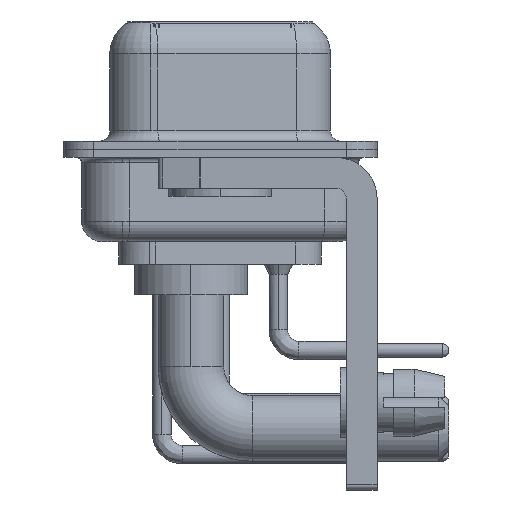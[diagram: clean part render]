
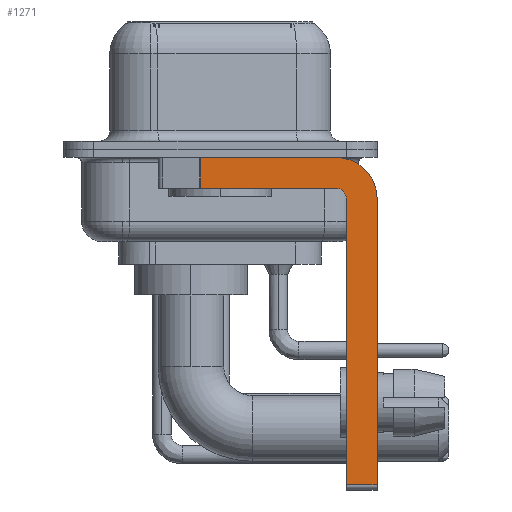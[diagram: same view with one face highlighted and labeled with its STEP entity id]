
A CAD part, left-side view. The second image highlights one B-rep face of the part: STEP entity #1271.
In plain terms, the highlighted planar face has unit normal (-1, 0, 0).
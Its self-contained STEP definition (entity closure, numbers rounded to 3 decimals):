
#229 = ORIENTED_EDGE ( 'NONE', *, *, #22137, .F. ) ;
#517 = DIRECTION ( 'NONE',  ( 0., 0., 1. ) ) ;
#1271 = ADVANCED_FACE ( 'NONE', ( #22588 ), #27415, .F. ) ;
#1882 = ORIENTED_EDGE ( 'NONE', *, *, #24168, .T. ) ;
#2416 = EDGE_CURVE ( 'NONE', #10307, #3281, #25507, .T. ) ;
#2463 = DIRECTION ( 'NONE',  ( 0., 0., -1. ) ) ;
#2919 = ORIENTED_EDGE ( 'NONE', *, *, #3153, .F. ) ;
#3153 = EDGE_CURVE ( 'NONE', #4360, #13230, #18464, .T. ) ;
#3281 = VERTEX_POINT ( 'NONE', #10403 ) ;
#3462 = ORIENTED_EDGE ( 'NONE', *, *, #10106, .F. ) ;
#3526 = DIRECTION ( 'NONE',  ( -1., 0., 0. ) ) ;
#4246 = DIRECTION ( 'NONE',  ( 0., 0., -1. ) ) ;
#4360 = VERTEX_POINT ( 'NONE', #17540 ) ;
#5350 = DIRECTION ( 'NONE',  ( 0., -1., 0. ) ) ;
#5502 = VECTOR ( 'NONE', #13557, 1000. ) ;
#6138 = AXIS2_PLACEMENT_3D ( 'NONE', #22110, #17615, #10553 ) ;
#6994 = EDGE_LOOP ( 'NONE', ( #8027, #1882, #2919, #229, #3462, #15904, #24967, #16377 ) ) ;
#7611 = CARTESIAN_POINT ( 'NONE',  ( -2.9, 3., -0.4 ) ) ;
#8027 = ORIENTED_EDGE ( 'NONE', *, *, #10384, .F. ) ;
#9107 = CARTESIAN_POINT ( 'NONE',  ( -2.9, -6.15, -16.35 ) ) ;
#10106 = EDGE_CURVE ( 'NONE', #26981, #18680, #11628, .T. ) ;
#10307 = VERTEX_POINT ( 'NONE', #22043 ) ;
#10359 = EDGE_CURVE ( 'NONE', #30653, #10307, #19841, .T. ) ;
#10384 = EDGE_CURVE ( 'NONE', #18487, #30653, #17218, .T. ) ;
#10403 = CARTESIAN_POINT ( 'NONE',  ( -2.9, -7.65, -16.35 ) ) ;
#10553 = DIRECTION ( 'NONE',  ( 0., 0., -1. ) ) ;
#11628 = LINE ( 'NONE', #25754, #5502 ) ;
#13230 = VERTEX_POINT ( 'NONE', #29028 ) ;
#13351 = DIRECTION ( 'NONE',  ( 0., 1., 0. ) ) ;
#13557 = DIRECTION ( 'NONE',  ( 0., 0., 1. ) ) ;
#15904 = ORIENTED_EDGE ( 'NONE', *, *, #20538, .T. ) ;
#16348 = CARTESIAN_POINT ( 'NONE',  ( -2.9, -7.65, -2.4 ) ) ;
#16377 = ORIENTED_EDGE ( 'NONE', *, *, #10359, .F. ) ;
#16552 = LINE ( 'NONE', #26031, #20680 ) ;
#16585 = VECTOR ( 'NONE', #13351, 1000. ) ;
#16738 = CARTESIAN_POINT ( 'NONE',  ( -2.9, -5.65, -2.4 ) ) ;
#17218 = LINE ( 'NONE', #7611, #27044 ) ;
#17540 = CARTESIAN_POINT ( 'NONE',  ( -2.9, -5.65, -1.9 ) ) ;
#17615 = DIRECTION ( 'NONE',  ( 1., 0., 0. ) ) ;
#17762 = CARTESIAN_POINT ( 'NONE',  ( -2.9, 0.978, -0.4 ) ) ;
#18464 = LINE ( 'NONE', #30682, #16585 ) ;
#18487 = VERTEX_POINT ( 'NONE', #17762 ) ;
#18680 = VERTEX_POINT ( 'NONE', #30923 ) ;
#19841 = CIRCLE ( 'NONE', #25499, 2. ) ;
#20538 = EDGE_CURVE ( 'NONE', #26981, #3281, #16552, .T. ) ;
#20680 = VECTOR ( 'NONE', #20894, 1000. ) ;
#20894 = DIRECTION ( 'NONE',  ( 0., -1., 0. ) ) ;
#21267 = LINE ( 'NONE', #28009, #29607 ) ;
#22043 = CARTESIAN_POINT ( 'NONE',  ( -2.9, -7.65, -2.4 ) ) ;
#22110 = CARTESIAN_POINT ( 'NONE',  ( -2.9, -5.65, -2.4 ) ) ;
#22137 = EDGE_CURVE ( 'NONE', #18680, #4360, #24335, .T. ) ;
#22588 = FACE_OUTER_BOUND ( 'NONE', #6994, .T. ) ;
#23833 = AXIS2_PLACEMENT_3D ( 'NONE', #25520, #3526, #517 ) ;
#24168 = EDGE_CURVE ( 'NONE', #18487, #13230, #21267, .T. ) ;
#24335 = CIRCLE ( 'NONE', #23833, 0.5 ) ;
#24967 = ORIENTED_EDGE ( 'NONE', *, *, #2416, .F. ) ;
#25247 = CARTESIAN_POINT ( 'NONE',  ( -2.9, -5.65, -0.4 ) ) ;
#25499 = AXIS2_PLACEMENT_3D ( 'NONE', #16738, #31683, #2463 ) ;
#25507 = LINE ( 'NONE', #16348, #25684 ) ;
#25520 = CARTESIAN_POINT ( 'NONE',  ( -2.9, -5.65, -2.4 ) ) ;
#25684 = VECTOR ( 'NONE', #26137, 1000. ) ;
#25754 = CARTESIAN_POINT ( 'NONE',  ( -2.9, -6.15, -16.6 ) ) ;
#26031 = CARTESIAN_POINT ( 'NONE',  ( -2.9, -5.65, -16.35 ) ) ;
#26137 = DIRECTION ( 'NONE',  ( 0., 0., -1. ) ) ;
#26981 = VERTEX_POINT ( 'NONE', #9107 ) ;
#27044 = VECTOR ( 'NONE', #5350, 1000. ) ;
#27415 = PLANE ( 'NONE',  #6138 ) ;
#28009 = CARTESIAN_POINT ( 'NONE',  ( -2.9, 0.978, -1.9 ) ) ;
#29028 = CARTESIAN_POINT ( 'NONE',  ( -2.9, 0.978, -1.9 ) ) ;
#29607 = VECTOR ( 'NONE', #4246, 1000. ) ;
#30653 = VERTEX_POINT ( 'NONE', #25247 ) ;
#30682 = CARTESIAN_POINT ( 'NONE',  ( -2.9, -5.65, -1.9 ) ) ;
#30923 = CARTESIAN_POINT ( 'NONE',  ( -2.9, -6.15, -2.4 ) ) ;
#31683 = DIRECTION ( 'NONE',  ( 1., 0., 0. ) ) ;
